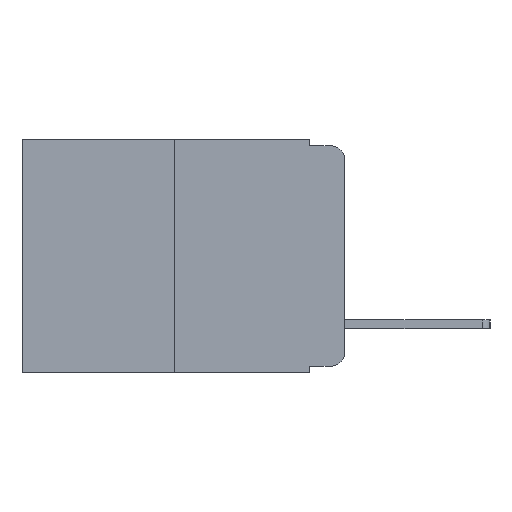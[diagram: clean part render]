
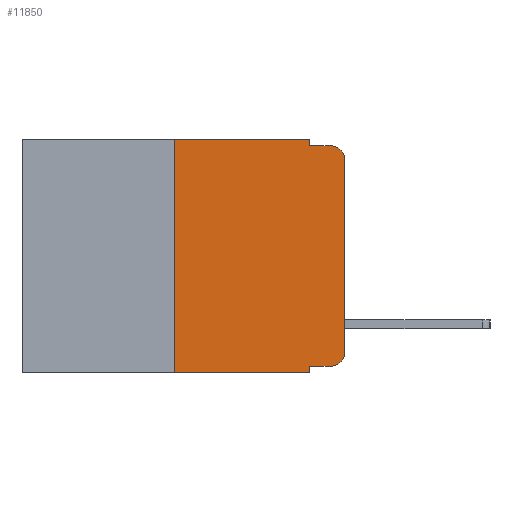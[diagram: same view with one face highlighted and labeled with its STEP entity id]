
A CAD part, left-side view. The second image highlights one B-rep face of the part: STEP entity #11850.
In plain terms, the highlighted planar face has unit normal (-1, 0, 0).
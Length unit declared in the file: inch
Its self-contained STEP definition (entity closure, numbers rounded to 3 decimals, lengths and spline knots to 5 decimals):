
#314 = CARTESIAN_POINT ( 'NONE',  ( 0., 0.473, -0.343 ) ) ;
#411 = EDGE_CURVE ( 'NONE', #12538, #5954, #13230, .T. ) ;
#758 = CARTESIAN_POINT ( 'NONE',  ( 0., 0.25, 0. ) ) ;
#1122 = CARTESIAN_POINT ( 'NONE',  ( 0., 0.02, -0.01 ) ) ;
#1134 = DIRECTION ( 'NONE',  ( 0., -1., 0. ) ) ;
#1349 = EDGE_CURVE ( 'NONE', #5994, #16716, #13200, .T. ) ;
#1496 = CARTESIAN_POINT ( 'NONE',  ( 0., 0.051, -0.333 ) ) ;
#1603 = LINE ( 'NONE', #758, #4838 ) ;
#2312 = AXIS2_PLACEMENT_3D ( 'NONE', #5815, #14923, #7185 ) ;
#2384 = PLANE ( 'NONE',  #6815 ) ;
#2402 = VECTOR ( 'NONE', #15035, 39.37008 ) ;
#2545 = EDGE_LOOP ( 'NONE', ( #3425, #4507, #4503, #9470, #6574, #12653, #11510, #3829, #12911, #7641 ) ) ;
#2915 = DIRECTION ( 'NONE',  ( 0., -1., 0. ) ) ;
#2940 = DIRECTION ( 'NONE',  ( -1., 0., 0. ) ) ;
#3107 = LINE ( 'NONE', #12482, #17017 ) ;
#3425 = ORIENTED_EDGE ( 'NONE', *, *, #15941, .T. ) ;
#3750 = DIRECTION ( 'NONE',  ( 1., 0., 0. ) ) ;
#3829 = ORIENTED_EDGE ( 'NONE', *, *, #1349, .F. ) ;
#4359 = CARTESIAN_POINT ( 'NONE',  ( 0., 0., -0.313 ) ) ;
#4370 = EDGE_CURVE ( 'NONE', #5954, #14514, #5176, .T. ) ;
#4503 = ORIENTED_EDGE ( 'NONE', *, *, #4370, .F. ) ;
#4507 = ORIENTED_EDGE ( 'NONE', *, *, #16338, .T. ) ;
#4584 = DIRECTION ( 'NONE',  ( 0., 0., 1. ) ) ;
#4751 = FACE_OUTER_BOUND ( 'NONE', #2545, .T. ) ;
#4838 = VECTOR ( 'NONE', #8886, 39.37008 ) ;
#5042 = VECTOR ( 'NONE', #2915, 39.37008 ) ;
#5047 = DIRECTION ( 'NONE',  ( 0., 0., -1. ) ) ;
#5176 = LINE ( 'NONE', #14434, #8327 ) ;
#5335 = CARTESIAN_POINT ( 'NONE',  ( 0., 0.051, 0. ) ) ;
#5458 = LINE ( 'NONE', #1496, #5042 ) ;
#5548 = CARTESIAN_POINT ( 'NONE',  ( 0., 0.051, -0.01 ) ) ;
#5815 = CARTESIAN_POINT ( 'NONE',  ( 0., 0.02, -0.313 ) ) ;
#5954 = VERTEX_POINT ( 'NONE', #5548 ) ;
#5994 = VERTEX_POINT ( 'NONE', #10887 ) ;
#6310 = VECTOR ( 'NONE', #5047, 39.37008 ) ;
#6401 = CARTESIAN_POINT ( 'NONE',  ( 0., 0., -0.03 ) ) ;
#6453 = EDGE_CURVE ( 'NONE', #13291, #7074, #12138, .T. ) ;
#6458 = LINE ( 'NONE', #314, #2402 ) ;
#6574 = ORIENTED_EDGE ( 'NONE', *, *, #10672, .F. ) ;
#6699 = CARTESIAN_POINT ( 'NONE',  ( 0., 0.25, 0. ) ) ;
#6815 = AXIS2_PLACEMENT_3D ( 'NONE', #11667, #3750, #12965 ) ;
#7074 = VERTEX_POINT ( 'NONE', #4359 ) ;
#7185 = DIRECTION ( 'NONE',  ( 0., 0., -1. ) ) ;
#7440 = AXIS2_PLACEMENT_3D ( 'NONE', #10879, #2940, #12186 ) ;
#7641 = ORIENTED_EDGE ( 'NONE', *, *, #6453, .T. ) ;
#7756 = VERTEX_POINT ( 'NONE', #8450 ) ;
#8327 = VECTOR ( 'NONE', #1134, 39.37008 ) ;
#8450 = CARTESIAN_POINT ( 'NONE',  ( 0., 0.25, -0.343 ) ) ;
#8886 = DIRECTION ( 'NONE',  ( 0., 0., 1. ) ) ;
#9470 = ORIENTED_EDGE ( 'NONE', *, *, #411, .F. ) ;
#9794 = VECTOR ( 'NONE', #13938, 39.37008 ) ;
#10630 = CARTESIAN_POINT ( 'NONE',  ( 0., 0.051, -0.343 ) ) ;
#10672 = EDGE_CURVE ( 'NONE', #10689, #12538, #14087, .T. ) ;
#10689 = VERTEX_POINT ( 'NONE', #6699 ) ;
#10879 = CARTESIAN_POINT ( 'NONE',  ( 0., 0.02, -0.03 ) ) ;
#10887 = CARTESIAN_POINT ( 'NONE',  ( 0., 0.051, -0.333 ) ) ;
#11510 = ORIENTED_EDGE ( 'NONE', *, *, #12224, .T. ) ;
#11667 = CARTESIAN_POINT ( 'NONE',  ( 0., 0.473, 0. ) ) ;
#11706 = CARTESIAN_POINT ( 'NONE',  ( 0., 0.051, 0. ) ) ;
#11821 = DIRECTION ( 'NONE',  ( 0., -1., 0. ) ) ;
#11850 = ADVANCED_FACE ( 'NONE', ( #4751 ), #2384, .F. ) ;
#12138 = CIRCLE ( 'NONE', #2312, 0.02 ) ;
#12186 = DIRECTION ( 'NONE',  ( 0., 0., -1. ) ) ;
#12224 = EDGE_CURVE ( 'NONE', #7756, #16716, #6458, .T. ) ;
#12411 = CARTESIAN_POINT ( 'NONE',  ( 0., 0.02, -0.333 ) ) ;
#12482 = CARTESIAN_POINT ( 'NONE',  ( 0., 0., 0. ) ) ;
#12538 = VERTEX_POINT ( 'NONE', #17142 ) ;
#12653 = ORIENTED_EDGE ( 'NONE', *, *, #15011, .F. ) ;
#12911 = ORIENTED_EDGE ( 'NONE', *, *, #15238, .T. ) ;
#12922 = VERTEX_POINT ( 'NONE', #6401 ) ;
#12965 = DIRECTION ( 'NONE',  ( 0., 0., -1. ) ) ;
#13200 = LINE ( 'NONE', #5335, #6310 ) ;
#13230 = LINE ( 'NONE', #11706, #9794 ) ;
#13291 = VERTEX_POINT ( 'NONE', #12411 ) ;
#13670 = VECTOR ( 'NONE', #11821, 39.37008 ) ;
#13938 = DIRECTION ( 'NONE',  ( 0., 0., -1. ) ) ;
#14087 = LINE ( 'NONE', #15697, #13670 ) ;
#14434 = CARTESIAN_POINT ( 'NONE',  ( 0., 0.051, -0.01 ) ) ;
#14514 = VERTEX_POINT ( 'NONE', #1122 ) ;
#14812 = CIRCLE ( 'NONE', #7440, 0.02 ) ;
#14923 = DIRECTION ( 'NONE',  ( -1., 0., 0. ) ) ;
#15011 = EDGE_CURVE ( 'NONE', #7756, #10689, #1603, .T. ) ;
#15035 = DIRECTION ( 'NONE',  ( 0., -1., 0. ) ) ;
#15238 = EDGE_CURVE ( 'NONE', #5994, #13291, #5458, .T. ) ;
#15697 = CARTESIAN_POINT ( 'NONE',  ( 0., 0.473, 0. ) ) ;
#15941 = EDGE_CURVE ( 'NONE', #7074, #12922, #3107, .T. ) ;
#16338 = EDGE_CURVE ( 'NONE', #12922, #14514, #14812, .T. ) ;
#16716 = VERTEX_POINT ( 'NONE', #10630 ) ;
#17017 = VECTOR ( 'NONE', #4584, 39.37008 ) ;
#17142 = CARTESIAN_POINT ( 'NONE',  ( 0., 0.051, 0. ) ) ;
